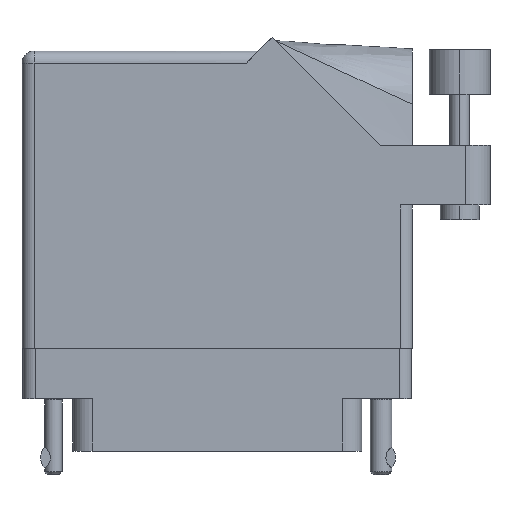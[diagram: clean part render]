
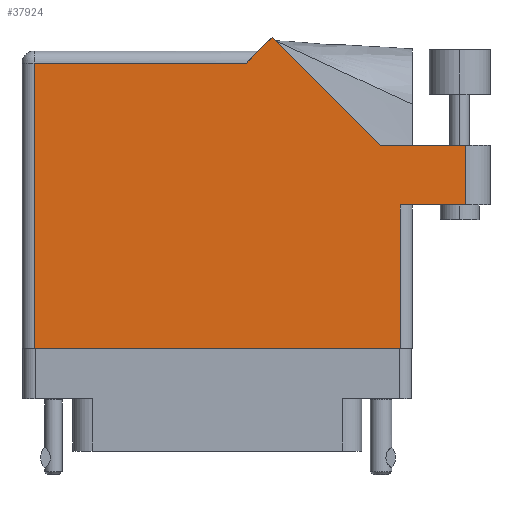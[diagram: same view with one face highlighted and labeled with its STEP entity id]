
A CAD part, front view. The second image highlights one B-rep face of the part: STEP entity #37924.
In plain terms, the highlighted face is planar.
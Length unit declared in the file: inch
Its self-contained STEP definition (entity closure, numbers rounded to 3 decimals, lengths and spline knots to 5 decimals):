
#1056 = CARTESIAN_POINT ( 'NONE',  ( 1.28771, 1.60071, 0. ) ) ;
#1072 = EDGE_CURVE ( 'NONE', #18391, #10691, #16296, .T. ) ;
#1143 = EDGE_LOOP ( 'NONE', ( #10168, #6694, #4183, #40539, #14973, #43649, #18537, #44048, #31971 ) ) ;
#1230 = CARTESIAN_POINT ( 'NONE',  ( 0.062, 1.468, 0. ) ) ;
#2165 = LINE ( 'NONE', #39801, #4504 ) ;
#2745 = DIRECTION ( 'NONE',  ( 0., 1., 0. ) ) ;
#3917 = CARTESIAN_POINT ( 'NONE',  ( 0., 0., 0. ) ) ;
#4183 = ORIENTED_EDGE ( 'NONE', *, *, #44970, .T. ) ;
#4492 = VERTEX_POINT ( 'NONE', #29159 ) ;
#4504 = VECTOR ( 'NONE', #21598, 39.37008 ) ;
#5318 = VECTOR ( 'NONE', #18669, 39.37008 ) ;
#6452 = VERTEX_POINT ( 'NONE', #41144 ) ;
#6694 = ORIENTED_EDGE ( 'NONE', *, *, #24234, .T. ) ;
#8252 = LINE ( 'NONE', #34322, #33834 ) ;
#8350 = EDGE_CURVE ( 'NONE', #10691, #43661, #39940, .T. ) ;
#9465 = CARTESIAN_POINT ( 'NONE',  ( 2.01, 0.737, 0. ) ) ;
#9837 = DIRECTION ( 'NONE',  ( 0., -1., 0. ) ) ;
#9946 = LINE ( 'NONE', #45106, #5318 ) ;
#10168 = ORIENTED_EDGE ( 'NONE', *, *, #43363, .T. ) ;
#10213 = VECTOR ( 'NONE', #42577, 39.37008 ) ;
#10691 = VERTEX_POINT ( 'NONE', #45923 ) ;
#12007 = VECTOR ( 'NONE', #12490, 39.37008 ) ;
#12490 = DIRECTION ( 'NONE',  ( 0., 1., 0. ) ) ;
#13174 = CARTESIAN_POINT ( 'NONE',  ( 1.84442, 1.044, 0. ) ) ;
#14973 = ORIENTED_EDGE ( 'NONE', *, *, #23443, .T. ) ;
#15038 = CARTESIAN_POINT ( 'NONE',  ( 0., 1.53, 0. ) ) ;
#16296 = LINE ( 'NONE', #24658, #33115 ) ;
#16628 = LINE ( 'NONE', #13174, #10213 ) ;
#18067 = EDGE_CURVE ( 'NONE', #20904, #18391, #8252, .T. ) ;
#18391 = VERTEX_POINT ( 'NONE', #1230 ) ;
#18537 = ORIENTED_EDGE ( 'NONE', *, *, #1072, .T. ) ;
#18669 = DIRECTION ( 'NONE',  ( -1., 0., 0. ) ) ;
#19657 = VERTEX_POINT ( 'NONE', #38542 ) ;
#20904 = VERTEX_POINT ( 'NONE', #26401 ) ;
#21598 = DIRECTION ( 'NONE',  ( -0.707, -0.707, 0. ) ) ;
#22081 = CARTESIAN_POINT ( 'NONE',  ( 1.948, 0., 0. ) ) ;
#23443 = EDGE_CURVE ( 'NONE', #25294, #20904, #2165, .T. ) ;
#24089 = EDGE_CURVE ( 'NONE', #45964, #25294, #16628, .T. ) ;
#24234 = EDGE_CURVE ( 'NONE', #6452, #19657, #42210, .T. ) ;
#24480 = EDGE_CURVE ( 'NONE', #43661, #4492, #46798, .T. ) ;
#24658 = CARTESIAN_POINT ( 'NONE',  ( 0.062, 0., 0. ) ) ;
#25152 = AXIS2_PLACEMENT_3D ( 'NONE', #15038, #44900, #26447 ) ;
#25294 = VERTEX_POINT ( 'NONE', #1056 ) ;
#25360 = VECTOR ( 'NONE', #2745, 39.37008 ) ;
#26401 = CARTESIAN_POINT ( 'NONE',  ( 1.155, 1.468, 0. ) ) ;
#26447 = DIRECTION ( 'NONE',  ( -1., 0., 0. ) ) ;
#27034 = DIRECTION ( 'NONE',  ( -1., 0., 0. ) ) ;
#29159 = CARTESIAN_POINT ( 'NONE',  ( 1.948, 0.737, 0. ) ) ;
#31971 = ORIENTED_EDGE ( 'NONE', *, *, #24480, .T. ) ;
#33115 = VECTOR ( 'NONE', #9837, 39.37008 ) ;
#33834 = VECTOR ( 'NONE', #27034, 39.37008 ) ;
#34322 = CARTESIAN_POINT ( 'NONE',  ( 0., 1.468, 0. ) ) ;
#34759 = CARTESIAN_POINT ( 'NONE',  ( 1.948, 0.737, 0. ) ) ;
#35616 = DIRECTION ( 'NONE',  ( 1., 0., 0. ) ) ;
#36640 = FACE_OUTER_BOUND ( 'NONE', #1143, .T. ) ;
#37410 = DIRECTION ( 'NONE',  ( 1., 0., 0. ) ) ;
#37924 = ADVANCED_FACE ( 'NONE', ( #36640 ), #44579, .F. ) ;
#38252 = VECTOR ( 'NONE', #37410, 39.37008 ) ;
#38542 = CARTESIAN_POINT ( 'NONE',  ( 2.285, 1.044, 0. ) ) ;
#38911 = CARTESIAN_POINT ( 'NONE',  ( 1.84442, 1.044, 0. ) ) ;
#39798 = CARTESIAN_POINT ( 'NONE',  ( 2.285, 1.044, 0. ) ) ;
#39801 = CARTESIAN_POINT ( 'NONE',  ( 1.217, 1.53, 0. ) ) ;
#39940 = LINE ( 'NONE', #3917, #38252 ) ;
#40539 = ORIENTED_EDGE ( 'NONE', *, *, #24089, .T. ) ;
#41144 = CARTESIAN_POINT ( 'NONE',  ( 2.285, 0.737, 0. ) ) ;
#41483 = VECTOR ( 'NONE', #35616, 39.37008 ) ;
#42210 = LINE ( 'NONE', #39798, #25360 ) ;
#42577 = DIRECTION ( 'NONE',  ( -0.707, 0.707, 0. ) ) ;
#43206 = LINE ( 'NONE', #9465, #41483 ) ;
#43363 = EDGE_CURVE ( 'NONE', #4492, #6452, #43206, .T. ) ;
#43649 = ORIENTED_EDGE ( 'NONE', *, *, #18067, .T. ) ;
#43661 = VERTEX_POINT ( 'NONE', #22081 ) ;
#44048 = ORIENTED_EDGE ( 'NONE', *, *, #8350, .T. ) ;
#44579 = PLANE ( 'NONE',  #25152 ) ;
#44900 = DIRECTION ( 'NONE',  ( 0., 0., -1. ) ) ;
#44970 = EDGE_CURVE ( 'NONE', #19657, #45964, #9946, .T. ) ;
#45106 = CARTESIAN_POINT ( 'NONE',  ( 2.41, 1.044, 0. ) ) ;
#45923 = CARTESIAN_POINT ( 'NONE',  ( 0.062, 0., 0. ) ) ;
#45964 = VERTEX_POINT ( 'NONE', #38911 ) ;
#46798 = LINE ( 'NONE', #34759, #12007 ) ;
